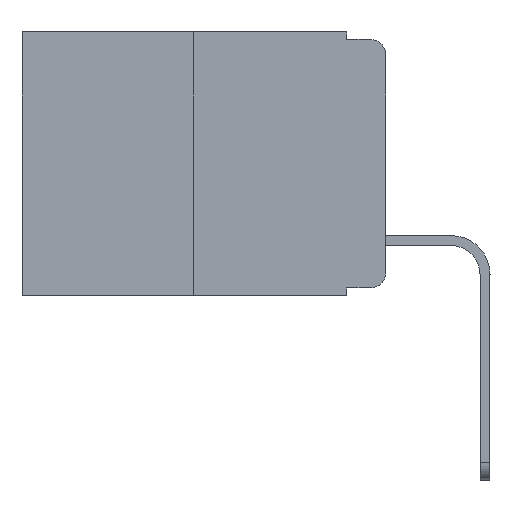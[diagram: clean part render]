
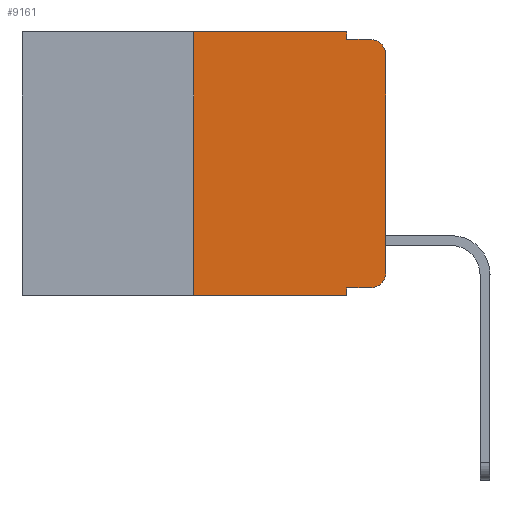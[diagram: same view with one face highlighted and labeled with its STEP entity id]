
A CAD part, left-side view. The second image highlights one B-rep face of the part: STEP entity #9161.
In plain terms, the highlighted planar face has unit normal (-1, 0, 0).
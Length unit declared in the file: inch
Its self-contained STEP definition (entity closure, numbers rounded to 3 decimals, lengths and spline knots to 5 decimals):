
#444 = CARTESIAN_POINT ( 'NONE',  ( 0., 0.25, -0.343 ) ) ;
#1016 = VERTEX_POINT ( 'NONE', #11359 ) ;
#1026 = DIRECTION ( 'NONE',  ( 0., -1., 0. ) ) ;
#1087 = DIRECTION ( 'NONE',  ( 0., 0., -1. ) ) ;
#1524 = CARTESIAN_POINT ( 'NONE',  ( 0., 0.051, -0.333 ) ) ;
#1603 = DIRECTION ( 'NONE',  ( -1., 0., 0. ) ) ;
#1909 = ORIENTED_EDGE ( 'NONE', *, *, #15020, .T. ) ;
#2267 = CARTESIAN_POINT ( 'NONE',  ( 0., 0.25, 0. ) ) ;
#2746 = DIRECTION ( 'NONE',  ( -1., 0., 0. ) ) ;
#2844 = VERTEX_POINT ( 'NONE', #444 ) ;
#2868 = DIRECTION ( 'NONE',  ( 0., 0., -1. ) ) ;
#3108 = ORIENTED_EDGE ( 'NONE', *, *, #5383, .T. ) ;
#3278 = LINE ( 'NONE', #15316, #16794 ) ;
#3478 = VERTEX_POINT ( 'NONE', #5637 ) ;
#3604 = CIRCLE ( 'NONE', #14603, 0.02 ) ;
#3842 = VECTOR ( 'NONE', #4107, 39.37008 ) ;
#4059 = CARTESIAN_POINT ( 'NONE',  ( 0., 0.051, -0.01 ) ) ;
#4107 = DIRECTION ( 'NONE',  ( 0., -1., 0. ) ) ;
#4378 = VERTEX_POINT ( 'NONE', #7534 ) ;
#4736 = CARTESIAN_POINT ( 'NONE',  ( 0., 0.051, -0.01 ) ) ;
#4936 = CARTESIAN_POINT ( 'NONE',  ( 0., 0.473, -0.343 ) ) ;
#5056 = ORIENTED_EDGE ( 'NONE', *, *, #9206, .F. ) ;
#5250 = VECTOR ( 'NONE', #7378, 39.37008 ) ;
#5350 = CARTESIAN_POINT ( 'NONE',  ( 0., 0.02, -0.333 ) ) ;
#5383 = EDGE_CURVE ( 'NONE', #14481, #3478, #3604, .T. ) ;
#5459 = LINE ( 'NONE', #4736, #5250 ) ;
#5561 = EDGE_CURVE ( 'NONE', #11659, #3478, #5459, .T. ) ;
#5637 = CARTESIAN_POINT ( 'NONE',  ( 0., 0.02, -0.01 ) ) ;
#5670 = VECTOR ( 'NONE', #5944, 39.37008 ) ;
#5944 = DIRECTION ( 'NONE',  ( 0., 0., -1. ) ) ;
#6152 = ORIENTED_EDGE ( 'NONE', *, *, #15559, .T. ) ;
#6418 = PLANE ( 'NONE',  #9168 ) ;
#6573 = VERTEX_POINT ( 'NONE', #5350 ) ;
#6752 = ORIENTED_EDGE ( 'NONE', *, *, #16791, .F. ) ;
#6818 = ORIENTED_EDGE ( 'NONE', *, *, #5561, .F. ) ;
#6853 = VERTEX_POINT ( 'NONE', #2267 ) ;
#7378 = DIRECTION ( 'NONE',  ( 0., -1., 0. ) ) ;
#7478 = DIRECTION ( 'NONE',  ( 0., 0., 1. ) ) ;
#7534 = CARTESIAN_POINT ( 'NONE',  ( 0., 0., -0.313 ) ) ;
#7650 = ORIENTED_EDGE ( 'NONE', *, *, #9919, .F. ) ;
#7985 = LINE ( 'NONE', #1524, #14112 ) ;
#8112 = LINE ( 'NONE', #16653, #10356 ) ;
#8526 = EDGE_CURVE ( 'NONE', #4378, #14481, #3278, .T. ) ;
#8529 = VERTEX_POINT ( 'NONE', #8801 ) ;
#8742 = EDGE_CURVE ( 'NONE', #6573, #4378, #12501, .T. ) ;
#8801 = CARTESIAN_POINT ( 'NONE',  ( 0., 0.051, -0.343 ) ) ;
#9161 = ADVANCED_FACE ( 'NONE', ( #12490 ), #6418, .F. ) ;
#9168 = AXIS2_PLACEMENT_3D ( 'NONE', #12930, #10212, #14186 ) ;
#9206 = EDGE_CURVE ( 'NONE', #14536, #11659, #8112, .T. ) ;
#9235 = ORIENTED_EDGE ( 'NONE', *, *, #8526, .T. ) ;
#9306 = DIRECTION ( 'NONE',  ( 0., -1., 0. ) ) ;
#9919 = EDGE_CURVE ( 'NONE', #6853, #14536, #13067, .T. ) ;
#10212 = DIRECTION ( 'NONE',  ( 1., 0., 0. ) ) ;
#10356 = VECTOR ( 'NONE', #1087, 39.37008 ) ;
#11048 = EDGE_LOOP ( 'NONE', ( #9235, #3108, #6818, #5056, #7650, #16438, #1909, #6752, #6152, #12463 ) ) ;
#11198 = CARTESIAN_POINT ( 'NONE',  ( 0., 0.051, 0. ) ) ;
#11359 = CARTESIAN_POINT ( 'NONE',  ( 0., 0.051, -0.333 ) ) ;
#11659 = VERTEX_POINT ( 'NONE', #4059 ) ;
#11863 = DIRECTION ( 'NONE',  ( 0., 0., 1. ) ) ;
#12131 = CARTESIAN_POINT ( 'NONE',  ( 0., 0.02, -0.03 ) ) ;
#12463 = ORIENTED_EDGE ( 'NONE', *, *, #8742, .T. ) ;
#12488 = VECTOR ( 'NONE', #11863, 39.37008 ) ;
#12490 = FACE_OUTER_BOUND ( 'NONE', #11048, .T. ) ;
#12501 = CIRCLE ( 'NONE', #14101, 0.02 ) ;
#12930 = CARTESIAN_POINT ( 'NONE',  ( 0., 0.473, 0. ) ) ;
#12996 = CARTESIAN_POINT ( 'NONE',  ( 0., 0.25, 0. ) ) ;
#13067 = LINE ( 'NONE', #14582, #3842 ) ;
#13105 = VECTOR ( 'NONE', #1026, 39.37008 ) ;
#13361 = CARTESIAN_POINT ( 'NONE',  ( 0., 0.02, -0.313 ) ) ;
#13526 = LINE ( 'NONE', #4936, #13105 ) ;
#13684 = DIRECTION ( 'NONE',  ( 0., 0., -1. ) ) ;
#14101 = AXIS2_PLACEMENT_3D ( 'NONE', #13361, #2746, #2868 ) ;
#14112 = VECTOR ( 'NONE', #9306, 39.37008 ) ;
#14186 = DIRECTION ( 'NONE',  ( 0., 0., -1. ) ) ;
#14380 = CARTESIAN_POINT ( 'NONE',  ( 0., 0., -0.03 ) ) ;
#14481 = VERTEX_POINT ( 'NONE', #14380 ) ;
#14536 = VERTEX_POINT ( 'NONE', #15868 ) ;
#14582 = CARTESIAN_POINT ( 'NONE',  ( 0., 0.473, 0. ) ) ;
#14603 = AXIS2_PLACEMENT_3D ( 'NONE', #12131, #1603, #13684 ) ;
#15020 = EDGE_CURVE ( 'NONE', #2844, #8529, #13526, .T. ) ;
#15124 = EDGE_CURVE ( 'NONE', #2844, #6853, #15150, .T. ) ;
#15150 = LINE ( 'NONE', #12996, #12488 ) ;
#15277 = LINE ( 'NONE', #11198, #5670 ) ;
#15316 = CARTESIAN_POINT ( 'NONE',  ( 0., 0., 0. ) ) ;
#15559 = EDGE_CURVE ( 'NONE', #1016, #6573, #7985, .T. ) ;
#15868 = CARTESIAN_POINT ( 'NONE',  ( 0., 0.051, 0. ) ) ;
#16438 = ORIENTED_EDGE ( 'NONE', *, *, #15124, .F. ) ;
#16653 = CARTESIAN_POINT ( 'NONE',  ( 0., 0.051, 0. ) ) ;
#16791 = EDGE_CURVE ( 'NONE', #1016, #8529, #15277, .T. ) ;
#16794 = VECTOR ( 'NONE', #7478, 39.37008 ) ;
